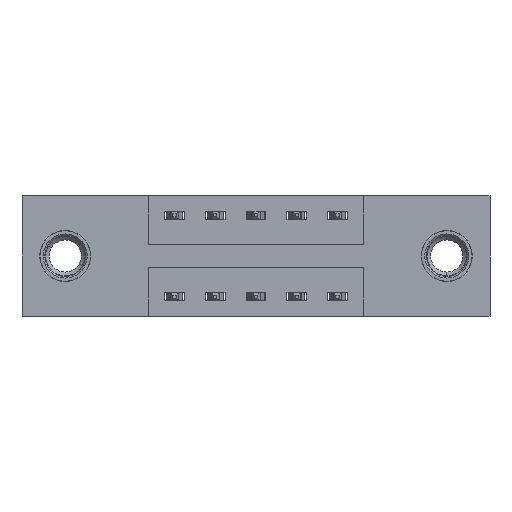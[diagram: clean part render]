
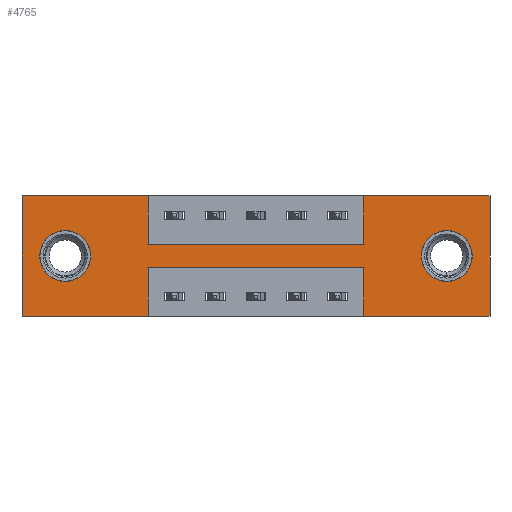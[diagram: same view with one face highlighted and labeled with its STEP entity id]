
A CAD part, front view. The second image highlights one B-rep face of the part: STEP entity #4765.
In plain terms, the highlighted planar face has unit normal (0, -1, 0).
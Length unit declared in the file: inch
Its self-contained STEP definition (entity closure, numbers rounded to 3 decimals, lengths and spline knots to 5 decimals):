
#18 = LINE ( 'NONE', #8741, #1947 ) ;
#19 = LINE ( 'NONE', #6556, #2262 ) ;
#59 = EDGE_CURVE ( 'NONE', #3457, #719, #4405, .T. ) ;
#107 = CARTESIAN_POINT ( 'NONE',  ( 0.3875, 0., -0.22 ) ) ;
#286 = DIRECTION ( 'NONE',  ( 0., 1., 0. ) ) ;
#336 = EDGE_CURVE ( 'NONE', #9138, #7303, #6316, .T. ) ;
#342 = CARTESIAN_POINT ( 'NONE',  ( 0., 0., -0.37 ) ) ;
#479 = EDGE_CURVE ( 'NONE', #7298, #7548, #3623, .T. ) ;
#593 = EDGE_CURVE ( 'NONE', #6775, #7298, #19, .T. ) ;
#605 = PLANE ( 'NONE',  #6219 ) ;
#719 = VERTEX_POINT ( 'NONE', #2543 ) ;
#854 = LINE ( 'NONE', #342, #5039 ) ;
#901 = CARTESIAN_POINT ( 'NONE',  ( 0.1325, 0., -0.107 ) ) ;
#1017 = VECTOR ( 'NONE', #7518, 39.37008 ) ;
#1025 = LINE ( 'NONE', #6118, #1435 ) ;
#1053 = EDGE_CURVE ( 'NONE', #7548, #7773, #3310, .T. ) ;
#1057 = VECTOR ( 'NONE', #7329, 39.37008 ) ;
#1148 = CARTESIAN_POINT ( 'NONE',  ( 0.3875, 0., -0.15 ) ) ;
#1313 = VECTOR ( 'NONE', #6886, 39.37008 ) ;
#1435 = VECTOR ( 'NONE', #9036, 39.37008 ) ;
#1566 = EDGE_CURVE ( 'NONE', #7481, #5578, #3830, .T. ) ;
#1631 = VECTOR ( 'NONE', #2439, 39.37008 ) ;
#1701 = ORIENTED_EDGE ( 'NONE', *, *, #479, .F. ) ;
#1947 = VECTOR ( 'NONE', #8028, 39.37008 ) ;
#2155 = VERTEX_POINT ( 'NONE', #3620 ) ;
#2178 = ORIENTED_EDGE ( 'NONE', *, *, #5638, .F. ) ;
#2262 = VECTOR ( 'NONE', #9452, 39.37008 ) ;
#2310 = ORIENTED_EDGE ( 'NONE', *, *, #6168, .F. ) ;
#2329 = ORIENTED_EDGE ( 'NONE', *, *, #8857, .T. ) ;
#2351 = VERTEX_POINT ( 'NONE', #8785 ) ;
#2417 = VECTOR ( 'NONE', #8076, 39.37008 ) ;
#2439 = DIRECTION ( 'NONE',  ( 0., 0., -1. ) ) ;
#2443 = EDGE_CURVE ( 'NONE', #2155, #9354, #8449, .T. ) ;
#2512 = CARTESIAN_POINT ( 'NONE',  ( 0.1325, 0., -0.185 ) ) ;
#2543 = CARTESIAN_POINT ( 'NONE',  ( 0.3875, 0., 0. ) ) ;
#2560 = EDGE_CURVE ( 'NONE', #7971, #2155, #3952, .T. ) ;
#2745 = DIRECTION ( 'NONE',  ( 1., 0., 0. ) ) ;
#2828 = DIRECTION ( 'NONE',  ( 0., 0., -1. ) ) ;
#2840 = VECTOR ( 'NONE', #5473, 39.37008 ) ;
#3055 = ORIENTED_EDGE ( 'NONE', *, *, #2560, .F. ) ;
#3310 = LINE ( 'NONE', #6869, #3522 ) ;
#3327 = EDGE_CURVE ( 'NONE', #7664, #6775, #1025, .T. ) ;
#3330 = DIRECTION ( 'NONE',  ( -1., 0., 0. ) ) ;
#3331 = ORIENTED_EDGE ( 'NONE', *, *, #6397, .F. ) ;
#3426 = DIRECTION ( 'NONE',  ( 0., 1., 0. ) ) ;
#3452 = CARTESIAN_POINT ( 'NONE',  ( 1.435, 0., -0.37 ) ) ;
#3457 = VERTEX_POINT ( 'NONE', #7931 ) ;
#3522 = VECTOR ( 'NONE', #7759, 39.37008 ) ;
#3541 = DIRECTION ( 'NONE',  ( 0., -1., 0. ) ) ;
#3605 = CARTESIAN_POINT ( 'NONE',  ( 0.3875, 0., -0.37 ) ) ;
#3620 = CARTESIAN_POINT ( 'NONE',  ( 1.435, 0., 0. ) ) ;
#3623 = LINE ( 'NONE', #5146, #2417 ) ;
#3697 = ORIENTED_EDGE ( 'NONE', *, *, #336, .F. ) ;
#3809 = VECTOR ( 'NONE', #2745, 39.37008 ) ;
#3816 = EDGE_LOOP ( 'NONE', ( #1701, #7207, #5169, #2178, #8753, #3055, #3331, #3697, #2310, #7275, #9102, #8552 ) ) ;
#3830 = CIRCLE ( 'NONE', #7805, 0.078 ) ;
#3952 = LINE ( 'NONE', #9120, #1313 ) ;
#4122 = DIRECTION ( 'NONE',  ( 0., 1., 0. ) ) ;
#4171 = DIRECTION ( 'NONE',  ( 0., 0., -1. ) ) ;
#4296 = CARTESIAN_POINT ( 'NONE',  ( 0.1325, 0., -0.185 ) ) ;
#4354 = EDGE_LOOP ( 'NONE', ( #8522, #5545 ) ) ;
#4405 = LINE ( 'NONE', #8848, #1057 ) ;
#4664 = CARTESIAN_POINT ( 'NONE',  ( 1.3025, 0., -0.185 ) ) ;
#4765 = ADVANCED_FACE ( 'NONE', ( #9285, #7194, #5543 ), #605, .T. ) ;
#5039 = VECTOR ( 'NONE', #3330, 39.37008 ) ;
#5146 = CARTESIAN_POINT ( 'NONE',  ( 0.3875, 0., -0.37 ) ) ;
#5169 = ORIENTED_EDGE ( 'NONE', *, *, #3327, .F. ) ;
#5299 = CARTESIAN_POINT ( 'NONE',  ( 1.0475, 0., 0. ) ) ;
#5322 = DIRECTION ( 'NONE',  ( 0., 0., -1. ) ) ;
#5431 = CIRCLE ( 'NONE', #9112, 0.078 ) ;
#5467 = CARTESIAN_POINT ( 'NONE',  ( 0.1325, 0., -0.263 ) ) ;
#5473 = DIRECTION ( 'NONE',  ( 0., 0., -1. ) ) ;
#5543 = FACE_OUTER_BOUND ( 'NONE', #3816, .T. ) ;
#5545 = ORIENTED_EDGE ( 'NONE', *, *, #1566, .T. ) ;
#5578 = VERTEX_POINT ( 'NONE', #901 ) ;
#5638 = EDGE_CURVE ( 'NONE', #9354, #7664, #854, .T. ) ;
#5681 = CARTESIAN_POINT ( 'NONE',  ( 0.3875, 0., -0.15 ) ) ;
#6007 = CARTESIAN_POINT ( 'NONE',  ( 1.0475, 0., -0.15 ) ) ;
#6033 = CIRCLE ( 'NONE', #7267, 0.078 ) ;
#6093 = EDGE_CURVE ( 'NONE', #6828, #2351, #6283, .T. ) ;
#6094 = LINE ( 'NONE', #9018, #1631 ) ;
#6118 = CARTESIAN_POINT ( 'NONE',  ( 1.0475, 0., -0.37 ) ) ;
#6168 = EDGE_CURVE ( 'NONE', #719, #9138, #6094, .T. ) ;
#6219 = AXIS2_PLACEMENT_3D ( 'NONE', #8473, #3541, #4171 ) ;
#6283 = CIRCLE ( 'NONE', #8418, 0.078 ) ;
#6316 = LINE ( 'NONE', #5681, #3809 ) ;
#6390 = CARTESIAN_POINT ( 'NONE',  ( 1.0475, 0., -0.37 ) ) ;
#6397 = EDGE_CURVE ( 'NONE', #7303, #7971, #8899, .T. ) ;
#6541 = CARTESIAN_POINT ( 'NONE',  ( 1.3025, 0., -0.185 ) ) ;
#6556 = CARTESIAN_POINT ( 'NONE',  ( 0.3875, 0., -0.22 ) ) ;
#6638 = EDGE_CURVE ( 'NONE', #7773, #3457, #18, .T. ) ;
#6681 = CARTESIAN_POINT ( 'NONE',  ( 0., 0., -0.37 ) ) ;
#6775 = VERTEX_POINT ( 'NONE', #8938 ) ;
#6828 = VERTEX_POINT ( 'NONE', #7415 ) ;
#6869 = CARTESIAN_POINT ( 'NONE',  ( 0., 0., -0.37 ) ) ;
#6886 = DIRECTION ( 'NONE',  ( 1., 0., 0. ) ) ;
#6977 = CARTESIAN_POINT ( 'NONE',  ( 1.435, 0., 0. ) ) ;
#7131 = DIRECTION ( 'NONE',  ( 0., 0., 1. ) ) ;
#7160 = EDGE_CURVE ( 'NONE', #5578, #7481, #5431, .T. ) ;
#7194 = FACE_BOUND ( 'NONE', #4354, .T. ) ;
#7207 = ORIENTED_EDGE ( 'NONE', *, *, #593, .F. ) ;
#7267 = AXIS2_PLACEMENT_3D ( 'NONE', #6541, #7867, #2828 ) ;
#7275 = ORIENTED_EDGE ( 'NONE', *, *, #59, .F. ) ;
#7276 = EDGE_LOOP ( 'NONE', ( #2329, #8562 ) ) ;
#7298 = VERTEX_POINT ( 'NONE', #107 ) ;
#7303 = VERTEX_POINT ( 'NONE', #6007 ) ;
#7329 = DIRECTION ( 'NONE',  ( 1., 0., 0. ) ) ;
#7415 = CARTESIAN_POINT ( 'NONE',  ( 1.3025, 0., -0.263 ) ) ;
#7481 = VERTEX_POINT ( 'NONE', #5467 ) ;
#7518 = DIRECTION ( 'NONE',  ( 0., 0., 1. ) ) ;
#7548 = VERTEX_POINT ( 'NONE', #3605 ) ;
#7581 = CARTESIAN_POINT ( 'NONE',  ( 1.0475, 0., 0. ) ) ;
#7664 = VERTEX_POINT ( 'NONE', #6390 ) ;
#7709 = DIRECTION ( 'NONE',  ( 0., 0., 1. ) ) ;
#7759 = DIRECTION ( 'NONE',  ( -1., 0., 0. ) ) ;
#7773 = VERTEX_POINT ( 'NONE', #6681 ) ;
#7805 = AXIS2_PLACEMENT_3D ( 'NONE', #2512, #4122, #7709 ) ;
#7867 = DIRECTION ( 'NONE',  ( 0., 1., 0. ) ) ;
#7931 = CARTESIAN_POINT ( 'NONE',  ( 0., 0., 0. ) ) ;
#7971 = VERTEX_POINT ( 'NONE', #7581 ) ;
#8028 = DIRECTION ( 'NONE',  ( 0., 0., 1. ) ) ;
#8076 = DIRECTION ( 'NONE',  ( 0., 0., -1. ) ) ;
#8418 = AXIS2_PLACEMENT_3D ( 'NONE', #4664, #286, #5322 ) ;
#8449 = LINE ( 'NONE', #6977, #2840 ) ;
#8473 = CARTESIAN_POINT ( 'NONE',  ( 0., 0., -0.37 ) ) ;
#8522 = ORIENTED_EDGE ( 'NONE', *, *, #7160, .T. ) ;
#8552 = ORIENTED_EDGE ( 'NONE', *, *, #1053, .F. ) ;
#8562 = ORIENTED_EDGE ( 'NONE', *, *, #6093, .T. ) ;
#8741 = CARTESIAN_POINT ( 'NONE',  ( 0., 0., 0. ) ) ;
#8753 = ORIENTED_EDGE ( 'NONE', *, *, #2443, .F. ) ;
#8785 = CARTESIAN_POINT ( 'NONE',  ( 1.3025, 0., -0.107 ) ) ;
#8848 = CARTESIAN_POINT ( 'NONE',  ( 0., 0., 0. ) ) ;
#8857 = EDGE_CURVE ( 'NONE', #2351, #6828, #6033, .T. ) ;
#8899 = LINE ( 'NONE', #5299, #1017 ) ;
#8938 = CARTESIAN_POINT ( 'NONE',  ( 1.0475, 0., -0.22 ) ) ;
#9018 = CARTESIAN_POINT ( 'NONE',  ( 0.3875, 0., 0. ) ) ;
#9036 = DIRECTION ( 'NONE',  ( 0., 0., 1. ) ) ;
#9102 = ORIENTED_EDGE ( 'NONE', *, *, #6638, .F. ) ;
#9112 = AXIS2_PLACEMENT_3D ( 'NONE', #4296, #3426, #7131 ) ;
#9120 = CARTESIAN_POINT ( 'NONE',  ( 0., 0., 0. ) ) ;
#9138 = VERTEX_POINT ( 'NONE', #1148 ) ;
#9285 = FACE_BOUND ( 'NONE', #7276, .T. ) ;
#9354 = VERTEX_POINT ( 'NONE', #3452 ) ;
#9452 = DIRECTION ( 'NONE',  ( -1., 0., 0. ) ) ;
